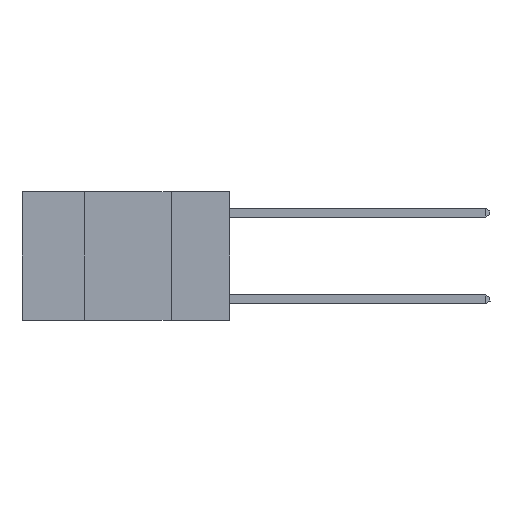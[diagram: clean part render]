
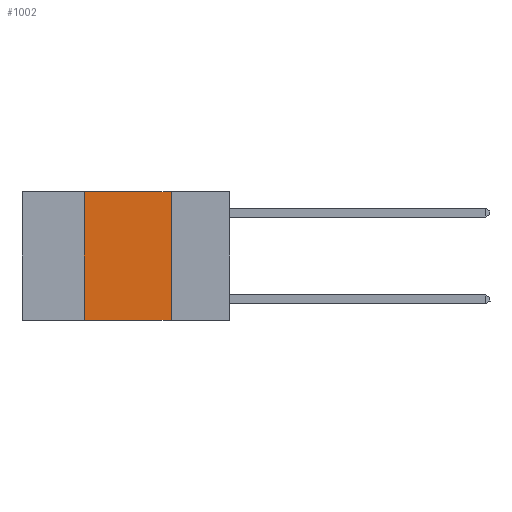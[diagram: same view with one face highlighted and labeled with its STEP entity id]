
A CAD part, left-side view. The second image highlights one B-rep face of the part: STEP entity #1002.
In plain terms, the highlighted planar face has unit normal (-1, 0, 0).
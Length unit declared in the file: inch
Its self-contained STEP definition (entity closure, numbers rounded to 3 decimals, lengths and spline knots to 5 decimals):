
#130 = DIRECTION ( 'NONE',  ( 0., 0., 1. ) ) ;
#396 = CARTESIAN_POINT ( 'NONE',  ( 0., 0.17, -0.37 ) ) ;
#1002 = ADVANCED_FACE ( 'NONE', ( #16533 ), #15649, .F. ) ;
#1735 = ORIENTED_EDGE ( 'NONE', *, *, #4223, .T. ) ;
#1916 = LINE ( 'NONE', #14576, #5586 ) ;
#2012 = CARTESIAN_POINT ( 'NONE',  ( 0., 0.6, 0. ) ) ;
#3040 = EDGE_CURVE ( 'NONE', #4378, #5963, #15872, .T. ) ;
#3549 = EDGE_CURVE ( 'NONE', #16384, #4378, #15015, .T. ) ;
#3686 = EDGE_CURVE ( 'NONE', #5963, #4739, #1916, .T. ) ;
#4223 = EDGE_CURVE ( 'NONE', #16384, #4739, #4697, .T. ) ;
#4268 = CARTESIAN_POINT ( 'NONE',  ( 0., 0.42, 0. ) ) ;
#4338 = AXIS2_PLACEMENT_3D ( 'NONE', #5563, #8174, #17186 ) ;
#4378 = VERTEX_POINT ( 'NONE', #4268 ) ;
#4697 = LINE ( 'NONE', #12242, #11592 ) ;
#4739 = VERTEX_POINT ( 'NONE', #396 ) ;
#5563 = CARTESIAN_POINT ( 'NONE',  ( 0., 0.6, 0. ) ) ;
#5586 = VECTOR ( 'NONE', #17572, 39.37008 ) ;
#5963 = VERTEX_POINT ( 'NONE', #10087 ) ;
#8174 = DIRECTION ( 'NONE',  ( 1., 0., 0. ) ) ;
#8657 = VECTOR ( 'NONE', #12710, 39.37008 ) ;
#8766 = DIRECTION ( 'NONE',  ( 0., -1., 0. ) ) ;
#10087 = CARTESIAN_POINT ( 'NONE',  ( 0., 0.17, 0. ) ) ;
#10680 = CARTESIAN_POINT ( 'NONE',  ( 0., 0.42, 0. ) ) ;
#10825 = ORIENTED_EDGE ( 'NONE', *, *, #3686, .F. ) ;
#10981 = CARTESIAN_POINT ( 'NONE',  ( 0., 0.42, -0.37 ) ) ;
#11407 = VECTOR ( 'NONE', #130, 39.37008 ) ;
#11550 = ORIENTED_EDGE ( 'NONE', *, *, #3040, .F. ) ;
#11592 = VECTOR ( 'NONE', #8766, 39.37008 ) ;
#12242 = CARTESIAN_POINT ( 'NONE',  ( 0., 0.6, -0.37 ) ) ;
#12640 = EDGE_LOOP ( 'NONE', ( #10825, #11550, #17570, #1735 ) ) ;
#12710 = DIRECTION ( 'NONE',  ( 0., -1., 0. ) ) ;
#14576 = CARTESIAN_POINT ( 'NONE',  ( 0., 0.17, 0. ) ) ;
#15015 = LINE ( 'NONE', #10680, #11407 ) ;
#15649 = PLANE ( 'NONE',  #4338 ) ;
#15872 = LINE ( 'NONE', #2012, #8657 ) ;
#16384 = VERTEX_POINT ( 'NONE', #10981 ) ;
#16533 = FACE_OUTER_BOUND ( 'NONE', #12640, .T. ) ;
#17186 = DIRECTION ( 'NONE',  ( 0., 0., -1. ) ) ;
#17570 = ORIENTED_EDGE ( 'NONE', *, *, #3549, .F. ) ;
#17572 = DIRECTION ( 'NONE',  ( 0., 0., -1. ) ) ;
